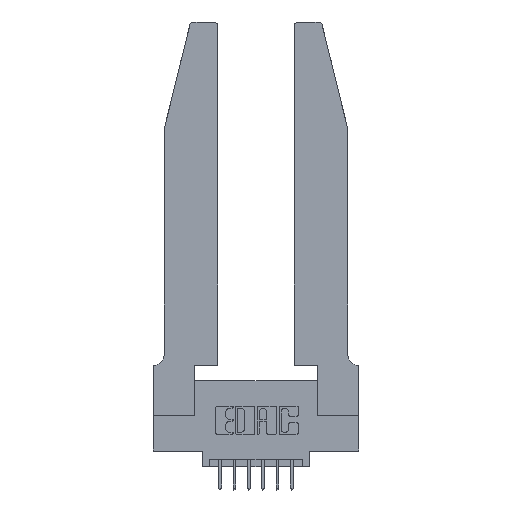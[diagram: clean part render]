
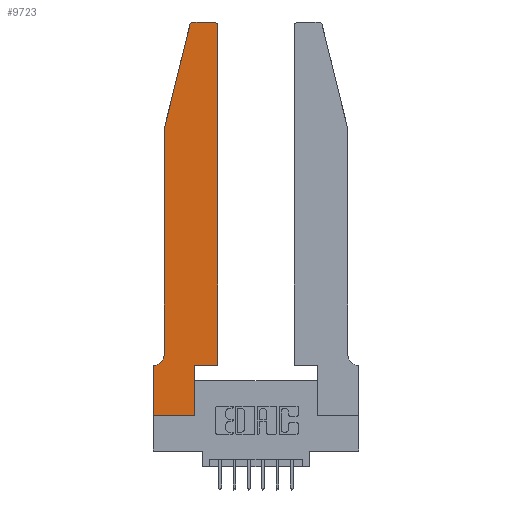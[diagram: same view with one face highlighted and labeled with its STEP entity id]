
A CAD part, top view. The second image highlights one B-rep face of the part: STEP entity #9723.
In plain terms, the highlighted planar face has unit normal (0, 0, 1).
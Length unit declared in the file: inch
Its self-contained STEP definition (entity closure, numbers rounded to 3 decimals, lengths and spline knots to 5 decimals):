
#246 = EDGE_CURVE ( 'NONE', #7778, #5044, #7551, .T. ) ;
#254 = DIRECTION ( 'NONE',  ( 0., 1., 0. ) ) ;
#384 = CARTESIAN_POINT ( 'NONE',  ( 0., 0.35, 0.37 ) ) ;
#478 = CARTESIAN_POINT ( 'NONE',  ( 0., 0., 0.37 ) ) ;
#818 = AXIS2_PLACEMENT_3D ( 'NONE', #13075, #6280, #2917 ) ;
#841 = CARTESIAN_POINT ( 'NONE',  ( 0.2865, 0.35, 0.37 ) ) ;
#939 = DIRECTION ( 'NONE',  ( 0., -1., 0. ) ) ;
#1163 = VERTEX_POINT ( 'NONE', #14039 ) ;
#1296 = LINE ( 'NONE', #5395, #1482 ) ;
#1307 = DIRECTION ( 'NONE',  ( 1., 0., 0. ) ) ;
#1482 = VECTOR ( 'NONE', #939, 39.37008 ) ;
#1620 = DIRECTION ( 'NONE',  ( 1., 0., 0. ) ) ;
#1639 = DIRECTION ( 'NONE',  ( -0.239, -0.971, 0. ) ) ;
#1669 = ORIENTED_EDGE ( 'NONE', *, *, #7955, .T. ) ;
#1673 = FACE_OUTER_BOUND ( 'NONE', #5229, .T. ) ;
#1682 = CARTESIAN_POINT ( 'NONE',  ( 0.4205, 2.72, 0.37 ) ) ;
#1701 = CIRCLE ( 'NONE', #818, 0.07 ) ;
#1865 = CARTESIAN_POINT ( 'NONE',  ( 0.25487, 2.72718, 0.37 ) ) ;
#2198 = CIRCLE ( 'NONE', #9137, 0.03 ) ;
#2827 = CARTESIAN_POINT ( 'NONE',  ( 0.4505, 0.35, 0.37 ) ) ;
#2917 = DIRECTION ( 'NONE',  ( -1., 0., 0. ) ) ;
#3018 = CIRCLE ( 'NONE', #14448, 0.03 ) ;
#3208 = LINE ( 'NONE', #8188, #5819 ) ;
#3292 = VERTEX_POINT ( 'NONE', #9436 ) ;
#3316 = CARTESIAN_POINT ( 'NONE',  ( 0., 0., 0.37 ) ) ;
#3557 = CARTESIAN_POINT ( 'NONE',  ( 0.284, 2.72, 0.37 ) ) ;
#3782 = LINE ( 'NONE', #13742, #8692 ) ;
#3910 = ORIENTED_EDGE ( 'NONE', *, *, #7795, .T. ) ;
#3938 = EDGE_CURVE ( 'NONE', #1163, #3292, #2198, .T. ) ;
#3952 = EDGE_CURVE ( 'NONE', #7555, #4699, #4856, .T. ) ;
#3971 = DIRECTION ( 'NONE',  ( 0., 0., 1. ) ) ;
#3998 = LINE ( 'NONE', #2827, #12226 ) ;
#4013 = CARTESIAN_POINT ( 'NONE',  ( 0.0755, 0.35, 0.37 ) ) ;
#4333 = VERTEX_POINT ( 'NONE', #384 ) ;
#4435 = LINE ( 'NONE', #9081, #13902 ) ;
#4563 = CARTESIAN_POINT ( 'NONE',  ( 0., 0.35, 0.37 ) ) ;
#4573 = VECTOR ( 'NONE', #8663, 39.37008 ) ;
#4620 = EDGE_CURVE ( 'NONE', #9625, #1163, #3998, .T. ) ;
#4699 = VERTEX_POINT ( 'NONE', #13956 ) ;
#4838 = CARTESIAN_POINT ( 'NONE',  ( 0.0055, 0.35, 0.37 ) ) ;
#4856 = LINE ( 'NONE', #10675, #13438 ) ;
#4909 = VERTEX_POINT ( 'NONE', #7029 ) ;
#5044 = VERTEX_POINT ( 'NONE', #14160 ) ;
#5078 = DIRECTION ( 'NONE',  ( 1., 0., 0. ) ) ;
#5229 = EDGE_LOOP ( 'NONE', ( #9994, #13052, #9083, #8116, #14193, #8030, #6633, #5367, #3910, #1669, #9149, #12454 ) ) ;
#5367 = ORIENTED_EDGE ( 'NONE', *, *, #246, .T. ) ;
#5395 = CARTESIAN_POINT ( 'NONE',  ( 0.0755, 2., 0.37 ) ) ;
#5819 = VECTOR ( 'NONE', #1620, 39.37008 ) ;
#5892 = EDGE_CURVE ( 'NONE', #4699, #13759, #1296, .T. ) ;
#6034 = EDGE_CURVE ( 'NONE', #4333, #7778, #3782, .T. ) ;
#6280 = DIRECTION ( 'NONE',  ( 0., 0., -1. ) ) ;
#6633 = ORIENTED_EDGE ( 'NONE', *, *, #6034, .T. ) ;
#6973 = DIRECTION ( 'NONE',  ( 0., 0., 1. ) ) ;
#7029 = CARTESIAN_POINT ( 'NONE',  ( 0.284, 2.75, 0.37 ) ) ;
#7220 = EDGE_CURVE ( 'NONE', #3292, #4909, #9542, .T. ) ;
#7252 = VERTEX_POINT ( 'NONE', #4838 ) ;
#7338 = DIRECTION ( 'NONE',  ( 0., 1., 0. ) ) ;
#7551 = LINE ( 'NONE', #478, #4573 ) ;
#7555 = VERTEX_POINT ( 'NONE', #1865 ) ;
#7605 = CARTESIAN_POINT ( 'NONE',  ( 0.4505, 0.35, 0.37 ) ) ;
#7770 = AXIS2_PLACEMENT_3D ( 'NONE', #4563, #10209, #1307 ) ;
#7778 = VERTEX_POINT ( 'NONE', #3316 ) ;
#7795 = EDGE_CURVE ( 'NONE', #5044, #12874, #4435, .T. ) ;
#7848 = EDGE_CURVE ( 'NONE', #4909, #7555, #3018, .T. ) ;
#7955 = EDGE_CURVE ( 'NONE', #12874, #9625, #3208, .T. ) ;
#7959 = DIRECTION ( 'NONE',  ( -1., 0., 0. ) ) ;
#8030 = ORIENTED_EDGE ( 'NONE', *, *, #9338, .T. ) ;
#8116 = ORIENTED_EDGE ( 'NONE', *, *, #5892, .T. ) ;
#8188 = CARTESIAN_POINT ( 'NONE',  ( 0.4505, 0.35, 0.37 ) ) ;
#8455 = DIRECTION ( 'NONE',  ( -1., 0., 0. ) ) ;
#8663 = DIRECTION ( 'NONE',  ( 1., 0., 0. ) ) ;
#8692 = VECTOR ( 'NONE', #10358, 39.37008 ) ;
#8991 = EDGE_CURVE ( 'NONE', #13759, #7252, #1701, .T. ) ;
#9081 = CARTESIAN_POINT ( 'NONE',  ( 0.2865, 0.35, 0.37 ) ) ;
#9083 = ORIENTED_EDGE ( 'NONE', *, *, #3952, .T. ) ;
#9137 = AXIS2_PLACEMENT_3D ( 'NONE', #1682, #3971, #5078 ) ;
#9149 = ORIENTED_EDGE ( 'NONE', *, *, #4620, .T. ) ;
#9258 = VECTOR ( 'NONE', #8455, 39.37008 ) ;
#9338 = EDGE_CURVE ( 'NONE', #7252, #4333, #12251, .T. ) ;
#9426 = CARTESIAN_POINT ( 'NONE',  ( 0.0755, 0.42, 0.37 ) ) ;
#9436 = CARTESIAN_POINT ( 'NONE',  ( 0.4205, 2.75, 0.37 ) ) ;
#9542 = LINE ( 'NONE', #12451, #10952 ) ;
#9625 = VERTEX_POINT ( 'NONE', #7605 ) ;
#9723 = ADVANCED_FACE ( 'NONE', ( #1673 ), #11256, .T. ) ;
#9994 = ORIENTED_EDGE ( 'NONE', *, *, #7220, .T. ) ;
#10209 = DIRECTION ( 'NONE',  ( 0., 0., 1. ) ) ;
#10358 = DIRECTION ( 'NONE',  ( 0., -1., 0. ) ) ;
#10675 = CARTESIAN_POINT ( 'NONE',  ( 0.0755, 2., 0.37 ) ) ;
#10952 = VECTOR ( 'NONE', #7959, 39.37008 ) ;
#11256 = PLANE ( 'NONE',  #7770 ) ;
#12226 = VECTOR ( 'NONE', #7338, 39.37008 ) ;
#12251 = LINE ( 'NONE', #4013, #9258 ) ;
#12451 = CARTESIAN_POINT ( 'NONE',  ( 0.2605, 2.75, 0.37 ) ) ;
#12454 = ORIENTED_EDGE ( 'NONE', *, *, #3938, .T. ) ;
#12874 = VERTEX_POINT ( 'NONE', #841 ) ;
#13052 = ORIENTED_EDGE ( 'NONE', *, *, #7848, .T. ) ;
#13075 = CARTESIAN_POINT ( 'NONE',  ( 0.0055, 0.42, 0.37 ) ) ;
#13438 = VECTOR ( 'NONE', #1639, 39.37008 ) ;
#13636 = DIRECTION ( 'NONE',  ( 1., 0., 0. ) ) ;
#13742 = CARTESIAN_POINT ( 'NONE',  ( 0., 0., 0.37 ) ) ;
#13759 = VERTEX_POINT ( 'NONE', #9426 ) ;
#13902 = VECTOR ( 'NONE', #254, 39.37008 ) ;
#13956 = CARTESIAN_POINT ( 'NONE',  ( 0.0755, 2., 0.37 ) ) ;
#14039 = CARTESIAN_POINT ( 'NONE',  ( 0.4505, 2.72, 0.37 ) ) ;
#14160 = CARTESIAN_POINT ( 'NONE',  ( 0.2865, 0., 0.37 ) ) ;
#14193 = ORIENTED_EDGE ( 'NONE', *, *, #8991, .T. ) ;
#14448 = AXIS2_PLACEMENT_3D ( 'NONE', #3557, #6973, #13636 ) ;
